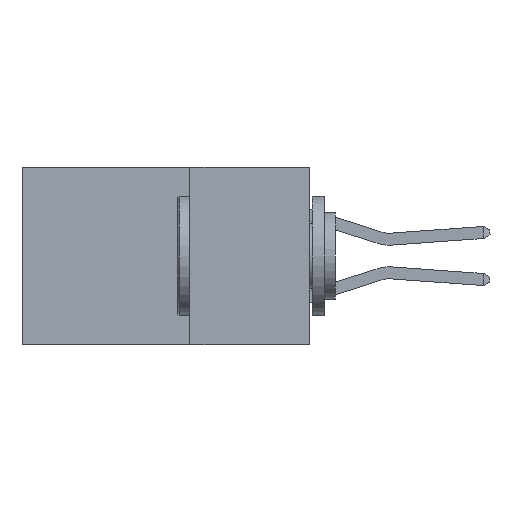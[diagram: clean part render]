
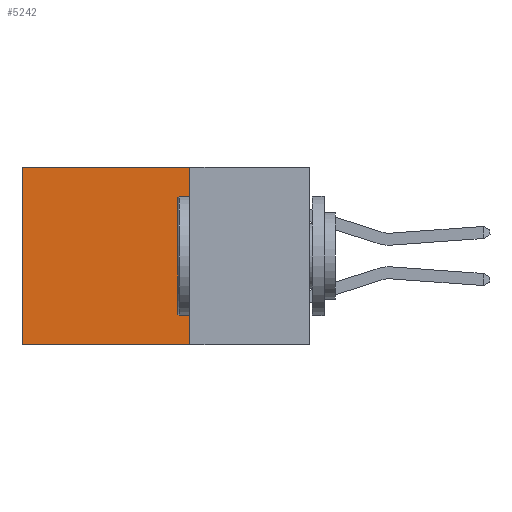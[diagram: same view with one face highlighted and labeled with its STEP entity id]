
A CAD part, left-side view. The second image highlights one B-rep face of the part: STEP entity #5242.
In plain terms, the highlighted planar face has unit normal (-1, 0, 0).
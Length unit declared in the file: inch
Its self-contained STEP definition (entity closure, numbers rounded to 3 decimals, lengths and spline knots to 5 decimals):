
#165 = CARTESIAN_POINT ( 'NONE',  ( 0.298, 0.6, 0. ) ) ;
#939 = EDGE_CURVE ( 'NONE', #5188, #7865, #3022, .T. ) ;
#2034 = DIRECTION ( 'NONE',  ( 0., 0., -1. ) ) ;
#3022 = LINE ( 'NONE', #165, #12978 ) ;
#3596 = ORIENTED_EDGE ( 'NONE', *, *, #939, .T. ) ;
#4213 = LINE ( 'NONE', #7016, #10740 ) ;
#4611 = VERTEX_POINT ( 'NONE', #5869 ) ;
#4831 = EDGE_CURVE ( 'NONE', #4611, #5188, #7359, .T. ) ;
#5188 = VERTEX_POINT ( 'NONE', #12002 ) ;
#5242 = ADVANCED_FACE ( 'NONE', ( #14995 ), #14005, .F. ) ;
#5869 = CARTESIAN_POINT ( 'NONE',  ( 0.298, 0.25, 0. ) ) ;
#7016 = CARTESIAN_POINT ( 'NONE',  ( 0.298, 0.25, 0. ) ) ;
#7145 = CARTESIAN_POINT ( 'NONE',  ( 0.298, 0.6, -0.37 ) ) ;
#7156 = DIRECTION ( 'NONE',  ( 0., 1., 0. ) ) ;
#7285 = DIRECTION ( 'NONE',  ( 1., 0., 0. ) ) ;
#7359 = LINE ( 'NONE', #10499, #13837 ) ;
#7865 = VERTEX_POINT ( 'NONE', #7145 ) ;
#8333 = DIRECTION ( 'NONE',  ( 0., 0., -1. ) ) ;
#8512 = EDGE_CURVE ( 'NONE', #4611, #11220, #4213, .T. ) ;
#9171 = EDGE_LOOP ( 'NONE', ( #3596, #16140, #10434, #13201 ) ) ;
#9812 = CARTESIAN_POINT ( 'NONE',  ( 0.298, 0.25, -0.37 ) ) ;
#10434 = ORIENTED_EDGE ( 'NONE', *, *, #8512, .F. ) ;
#10499 = CARTESIAN_POINT ( 'NONE',  ( 0.298, 0.25, 0. ) ) ;
#10740 = VECTOR ( 'NONE', #8333, 39.37008 ) ;
#11100 = CARTESIAN_POINT ( 'NONE',  ( 0.298, 0.25, -0.37 ) ) ;
#11220 = VERTEX_POINT ( 'NONE', #9812 ) ;
#12002 = CARTESIAN_POINT ( 'NONE',  ( 0.298, 0.6, 0. ) ) ;
#12018 = LINE ( 'NONE', #11100, #15370 ) ;
#12546 = EDGE_CURVE ( 'NONE', #11220, #7865, #12018, .T. ) ;
#12978 = VECTOR ( 'NONE', #16053, 39.37008 ) ;
#13085 = DIRECTION ( 'NONE',  ( 0., 1., 0. ) ) ;
#13201 = ORIENTED_EDGE ( 'NONE', *, *, #4831, .T. ) ;
#13837 = VECTOR ( 'NONE', #13085, 39.37008 ) ;
#14005 = PLANE ( 'NONE',  #16468 ) ;
#14073 = CARTESIAN_POINT ( 'NONE',  ( 0.298, 0.25, 0. ) ) ;
#14995 = FACE_OUTER_BOUND ( 'NONE', #9171, .T. ) ;
#15370 = VECTOR ( 'NONE', #7156, 39.37008 ) ;
#16053 = DIRECTION ( 'NONE',  ( 0., 0., -1. ) ) ;
#16140 = ORIENTED_EDGE ( 'NONE', *, *, #12546, .F. ) ;
#16468 = AXIS2_PLACEMENT_3D ( 'NONE', #14073, #7285, #2034 ) ;
